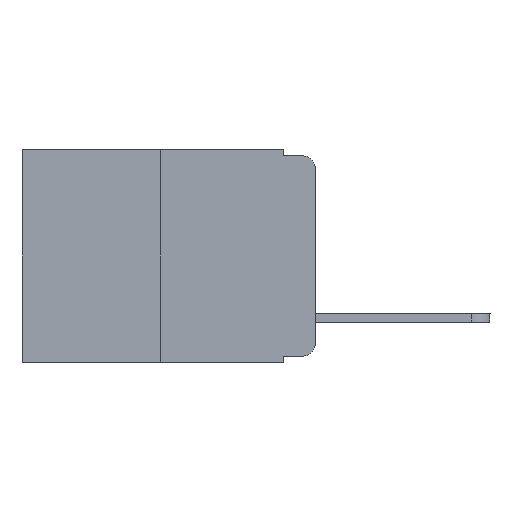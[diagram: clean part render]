
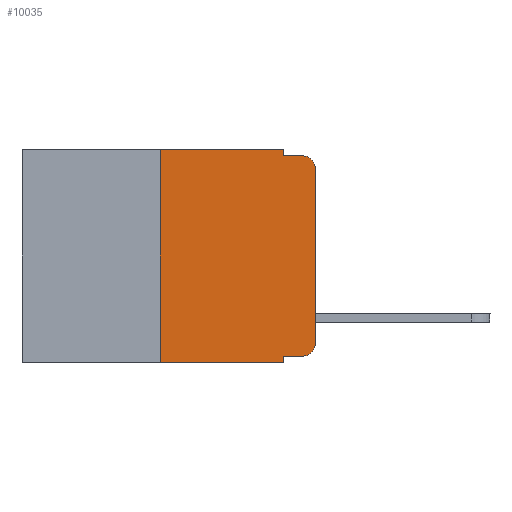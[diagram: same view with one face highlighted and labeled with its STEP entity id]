
A CAD part, left-side view. The second image highlights one B-rep face of the part: STEP entity #10035.
In plain terms, the highlighted planar face has unit normal (-1, 0, 0).
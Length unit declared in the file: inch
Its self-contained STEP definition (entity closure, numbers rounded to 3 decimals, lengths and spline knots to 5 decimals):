
#50 = AXIS2_PLACEMENT_3D ( 'NONE', #89, #16065, #5712 ) ;
#89 = CARTESIAN_POINT ( 'NONE',  ( 0., 0.02, -0.313 ) ) ;
#154 = VECTOR ( 'NONE', #6208, 39.37008 ) ;
#204 = CARTESIAN_POINT ( 'NONE',  ( 0., 0.02, -0.333 ) ) ;
#721 = CARTESIAN_POINT ( 'NONE',  ( 0., 0.02, -0.03 ) ) ;
#1258 = LINE ( 'NONE', #20762, #154 ) ;
#1359 = ORIENTED_EDGE ( 'NONE', *, *, #4840, .F. ) ;
#2353 = PLANE ( 'NONE',  #18846 ) ;
#2818 = DIRECTION ( 'NONE',  ( -1., 0., 0. ) ) ;
#3202 = CARTESIAN_POINT ( 'NONE',  ( 0., 0.25, -0.343 ) ) ;
#3633 = CARTESIAN_POINT ( 'NONE',  ( 0., 0.051, -0.333 ) ) ;
#4693 = CARTESIAN_POINT ( 'NONE',  ( 0., 0.02, -0.01 ) ) ;
#4695 = EDGE_CURVE ( 'NONE', #10148, #22107, #15869, .T. ) ;
#4840 = EDGE_CURVE ( 'NONE', #13705, #14558, #1258, .T. ) ;
#4860 = VECTOR ( 'NONE', #19451, 39.37008 ) ;
#4928 = DIRECTION ( 'NONE',  ( 1., 0., 0. ) ) ;
#5132 = CARTESIAN_POINT ( 'NONE',  ( 0., 0.473, -0.343 ) ) ;
#5712 = DIRECTION ( 'NONE',  ( 0., 0., -1. ) ) ;
#5747 = EDGE_CURVE ( 'NONE', #13705, #19100, #9151, .T. ) ;
#6208 = DIRECTION ( 'NONE',  ( 0., 0., -1. ) ) ;
#6597 = CARTESIAN_POINT ( 'NONE',  ( 0., 0.473, 0. ) ) ;
#6602 = LINE ( 'NONE', #22333, #9850 ) ;
#6936 = CARTESIAN_POINT ( 'NONE',  ( 0., 0.051, -0.333 ) ) ;
#6950 = DIRECTION ( 'NONE',  ( 0., 0., 1. ) ) ;
#6985 = ORIENTED_EDGE ( 'NONE', *, *, #15295, .F. ) ;
#7279 = CARTESIAN_POINT ( 'NONE',  ( 0., 0.051, 0. ) ) ;
#7748 = VERTEX_POINT ( 'NONE', #22505 ) ;
#8180 = ORIENTED_EDGE ( 'NONE', *, *, #19140, .T. ) ;
#8221 = CARTESIAN_POINT ( 'NONE',  ( 0., 0., -0.313 ) ) ;
#8713 = EDGE_CURVE ( 'NONE', #22107, #17329, #11349, .T. ) ;
#8779 = CARTESIAN_POINT ( 'NONE',  ( 0., 0.051, 0. ) ) ;
#9151 = LINE ( 'NONE', #6936, #10716 ) ;
#9535 = CARTESIAN_POINT ( 'NONE',  ( 0., 0.473, 0. ) ) ;
#9571 = CARTESIAN_POINT ( 'NONE',  ( 0., 0., -0.03 ) ) ;
#9850 = VECTOR ( 'NONE', #10361, 39.37008 ) ;
#10035 = ADVANCED_FACE ( 'NONE', ( #18451 ), #2353, .F. ) ;
#10051 = EDGE_CURVE ( 'NONE', #7748, #17329, #6602, .T. ) ;
#10148 = VERTEX_POINT ( 'NONE', #8221 ) ;
#10361 = DIRECTION ( 'NONE',  ( 0., -1., 0. ) ) ;
#10716 = VECTOR ( 'NONE', #19848, 39.37008 ) ;
#11301 = CARTESIAN_POINT ( 'NONE',  ( 0., 0.051, -0.343 ) ) ;
#11349 = CIRCLE ( 'NONE', #18848, 0.02 ) ;
#11779 = ORIENTED_EDGE ( 'NONE', *, *, #17681, .T. ) ;
#11873 = VECTOR ( 'NONE', #6950, 39.37008 ) ;
#12126 = ORIENTED_EDGE ( 'NONE', *, *, #8713, .T. ) ;
#12232 = ORIENTED_EDGE ( 'NONE', *, *, #18614, .F. ) ;
#13138 = VECTOR ( 'NONE', #17517, 39.37008 ) ;
#13158 = ORIENTED_EDGE ( 'NONE', *, *, #4695, .T. ) ;
#13705 = VERTEX_POINT ( 'NONE', #3633 ) ;
#13961 = LINE ( 'NONE', #8779, #18246 ) ;
#14558 = VERTEX_POINT ( 'NONE', #11301 ) ;
#15149 = DIRECTION ( 'NONE',  ( 0., 0., -1. ) ) ;
#15295 = EDGE_CURVE ( 'NONE', #17472, #7748, #13961, .T. ) ;
#15850 = LINE ( 'NONE', #6597, #13138 ) ;
#15869 = LINE ( 'NONE', #23040, #11873 ) ;
#15879 = VECTOR ( 'NONE', #22778, 39.37008 ) ;
#15961 = DIRECTION ( 'NONE',  ( 0., 0., -1. ) ) ;
#16065 = DIRECTION ( 'NONE',  ( -1., 0., 0. ) ) ;
#16145 = CIRCLE ( 'NONE', #50, 0.02 ) ;
#16578 = EDGE_LOOP ( 'NONE', ( #13158, #12126, #17759, #6985, #12232, #19133, #11779, #1359, #22094, #8180 ) ) ;
#17329 = VERTEX_POINT ( 'NONE', #4693 ) ;
#17472 = VERTEX_POINT ( 'NONE', #7279 ) ;
#17517 = DIRECTION ( 'NONE',  ( 0., -1., 0. ) ) ;
#17681 = EDGE_CURVE ( 'NONE', #22330, #14558, #21237, .T. ) ;
#17759 = ORIENTED_EDGE ( 'NONE', *, *, #10051, .F. ) ;
#18246 = VECTOR ( 'NONE', #15961, 39.37008 ) ;
#18451 = FACE_OUTER_BOUND ( 'NONE', #16578, .T. ) ;
#18553 = LINE ( 'NONE', #21010, #15879 ) ;
#18614 = EDGE_CURVE ( 'NONE', #22825, #17472, #15850, .T. ) ;
#18846 = AXIS2_PLACEMENT_3D ( 'NONE', #9535, #4928, #15149 ) ;
#18848 = AXIS2_PLACEMENT_3D ( 'NONE', #721, #2818, #20462 ) ;
#19100 = VERTEX_POINT ( 'NONE', #204 ) ;
#19133 = ORIENTED_EDGE ( 'NONE', *, *, #21257, .F. ) ;
#19140 = EDGE_CURVE ( 'NONE', #19100, #10148, #16145, .T. ) ;
#19451 = DIRECTION ( 'NONE',  ( 0., -1., 0. ) ) ;
#19848 = DIRECTION ( 'NONE',  ( 0., -1., 0. ) ) ;
#20462 = DIRECTION ( 'NONE',  ( 0., 0., -1. ) ) ;
#20762 = CARTESIAN_POINT ( 'NONE',  ( 0., 0.051, 0. ) ) ;
#21010 = CARTESIAN_POINT ( 'NONE',  ( 0., 0.25, 0. ) ) ;
#21237 = LINE ( 'NONE', #5132, #4860 ) ;
#21257 = EDGE_CURVE ( 'NONE', #22330, #22825, #18553, .T. ) ;
#21604 = CARTESIAN_POINT ( 'NONE',  ( 0., 0.25, 0. ) ) ;
#22094 = ORIENTED_EDGE ( 'NONE', *, *, #5747, .T. ) ;
#22107 = VERTEX_POINT ( 'NONE', #9571 ) ;
#22330 = VERTEX_POINT ( 'NONE', #3202 ) ;
#22333 = CARTESIAN_POINT ( 'NONE',  ( 0., 0.051, -0.01 ) ) ;
#22505 = CARTESIAN_POINT ( 'NONE',  ( 0., 0.051, -0.01 ) ) ;
#22778 = DIRECTION ( 'NONE',  ( 0., 0., 1. ) ) ;
#22825 = VERTEX_POINT ( 'NONE', #21604 ) ;
#23040 = CARTESIAN_POINT ( 'NONE',  ( 0., 0., 0. ) ) ;
